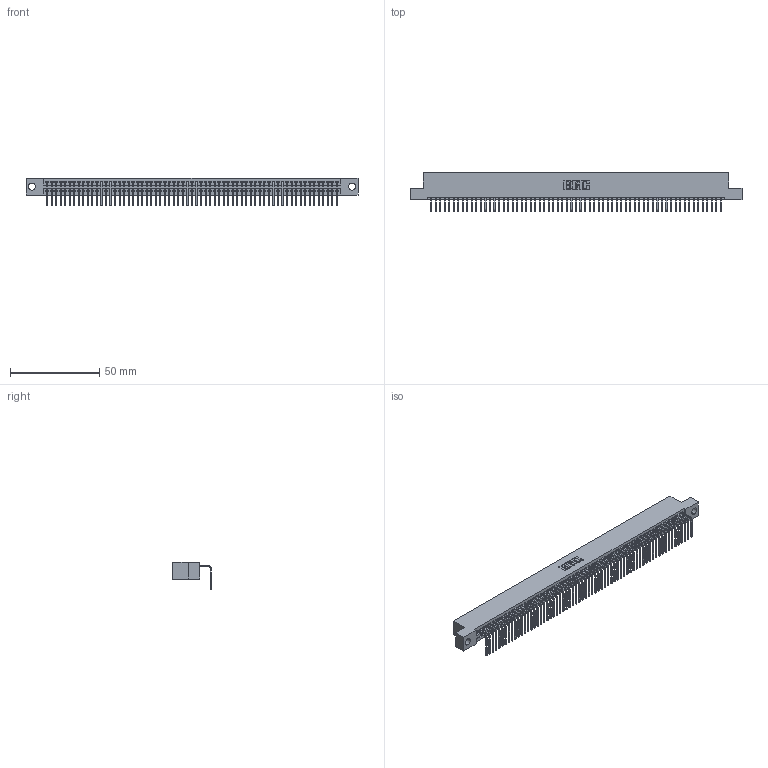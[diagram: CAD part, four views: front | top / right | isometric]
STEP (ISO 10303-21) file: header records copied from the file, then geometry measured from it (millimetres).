
FILE_DESCRIPTION (( 'STEP AP203' ), '1' );
FILE_NAME ('345-065-558-104.STEP', '2021-06-10T15:09:46', ( '' ), ( '' ), 'SwSTEP 2.0', 'SolidWorks 2020', '' );
FILE_SCHEMA (( 'CONFIG_CONTROL_DESIGN' ));
Length unit declared in the file: inch
Products named in the file (3): 345-292-001_558 Tail - 2; 345-065-558-104; 345 Part_Flush Mounting Lugs - 0.156 Dia-TI
Assembly tree (66 placements, depth 2):
  345-065-558-104
    345 Part_Flush Mounting Lugs - 0.156 Dia-TI
    345-292-001_558 Tail - 2  x65
Bounding box: 186.31 x 21.83 x 15.37 mm (x, y, z)
Volume: 17994.8 mm3; surface area: 25341.1 mm2
Topology: 66 solids, 66 shells, 4040 faces, 12207 edges, 8050 vertices
Faces by surface type: plane 2824, cylinder 1216
Entity records: 46327 total; most frequent: CARTESIAN_POINT 8033, ORIENTED_EDGE 8030, DIRECTION 6981, EDGE_CURVE 4015, VECTOR 3623, LINE 3623, VERTEX_POINT 2674, AXIS2_PLACEMENT_3D 1679
